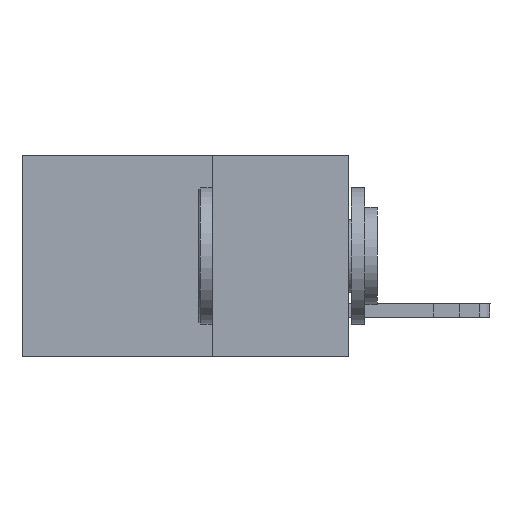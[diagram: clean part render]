
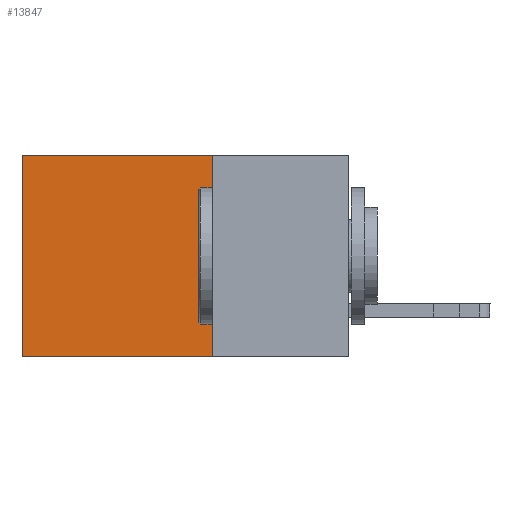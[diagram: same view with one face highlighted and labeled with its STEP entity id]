
A CAD part, left-side view. The second image highlights one B-rep face of the part: STEP entity #13847.
In plain terms, the highlighted planar face has unit normal (-1, 0, 0).
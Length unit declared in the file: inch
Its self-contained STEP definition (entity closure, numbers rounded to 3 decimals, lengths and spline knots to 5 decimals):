
#185 = EDGE_CURVE ( 'NONE', #2711, #7955, #4044, .T. ) ;
#1718 = CARTESIAN_POINT ( 'NONE',  ( 0.298, 0.25, 0. ) ) ;
#1945 = EDGE_CURVE ( 'NONE', #2686, #7955, #13658, .T. ) ;
#2686 = VERTEX_POINT ( 'NONE', #12677 ) ;
#2711 = VERTEX_POINT ( 'NONE', #11569 ) ;
#2788 = DIRECTION ( 'NONE',  ( 0., 1., 0. ) ) ;
#3374 = CARTESIAN_POINT ( 'NONE',  ( 0.298, 0.6, -0.37 ) ) ;
#4044 = LINE ( 'NONE', #12937, #9416 ) ;
#4311 = DIRECTION ( 'NONE',  ( 1., 0., 0. ) ) ;
#4393 = DIRECTION ( 'NONE',  ( 0., 0., -1. ) ) ;
#4505 = VECTOR ( 'NONE', #6202, 39.37008 ) ;
#4604 = LINE ( 'NONE', #1718, #7300 ) ;
#4899 = DIRECTION ( 'NONE',  ( 0., 1., 0. ) ) ;
#5034 = CARTESIAN_POINT ( 'NONE',  ( 0.298, 0.25, 0. ) ) ;
#5513 = EDGE_CURVE ( 'NONE', #10695, #2711, #4604, .T. ) ;
#6202 = DIRECTION ( 'NONE',  ( 0., 0., -1. ) ) ;
#6585 = AXIS2_PLACEMENT_3D ( 'NONE', #8509, #4311, #4393 ) ;
#7300 = VECTOR ( 'NONE', #2788, 39.37008 ) ;
#7449 = PLANE ( 'NONE',  #6585 ) ;
#7729 = EDGE_CURVE ( 'NONE', #10695, #2686, #11909, .T. ) ;
#7884 = VECTOR ( 'NONE', #4899, 39.37008 ) ;
#7911 = CARTESIAN_POINT ( 'NONE',  ( 0.298, 0.25, -0.37 ) ) ;
#7955 = VERTEX_POINT ( 'NONE', #3374 ) ;
#8509 = CARTESIAN_POINT ( 'NONE',  ( 0.298, 0.25, 0. ) ) ;
#9416 = VECTOR ( 'NONE', #9507, 39.37008 ) ;
#9507 = DIRECTION ( 'NONE',  ( 0., 0., -1. ) ) ;
#9664 = EDGE_LOOP ( 'NONE', ( #11110, #13575, #9692, #10278 ) ) ;
#9692 = ORIENTED_EDGE ( 'NONE', *, *, #7729, .F. ) ;
#10278 = ORIENTED_EDGE ( 'NONE', *, *, #5513, .T. ) ;
#10695 = VERTEX_POINT ( 'NONE', #11792 ) ;
#11110 = ORIENTED_EDGE ( 'NONE', *, *, #185, .T. ) ;
#11111 = FACE_OUTER_BOUND ( 'NONE', #9664, .T. ) ;
#11569 = CARTESIAN_POINT ( 'NONE',  ( 0.298, 0.6, 0. ) ) ;
#11792 = CARTESIAN_POINT ( 'NONE',  ( 0.298, 0.25, 0. ) ) ;
#11909 = LINE ( 'NONE', #5034, #4505 ) ;
#12677 = CARTESIAN_POINT ( 'NONE',  ( 0.298, 0.25, -0.37 ) ) ;
#12937 = CARTESIAN_POINT ( 'NONE',  ( 0.298, 0.6, 0. ) ) ;
#13575 = ORIENTED_EDGE ( 'NONE', *, *, #1945, .F. ) ;
#13658 = LINE ( 'NONE', #7911, #7884 ) ;
#13847 = ADVANCED_FACE ( 'NONE', ( #11111 ), #7449, .F. ) ;
